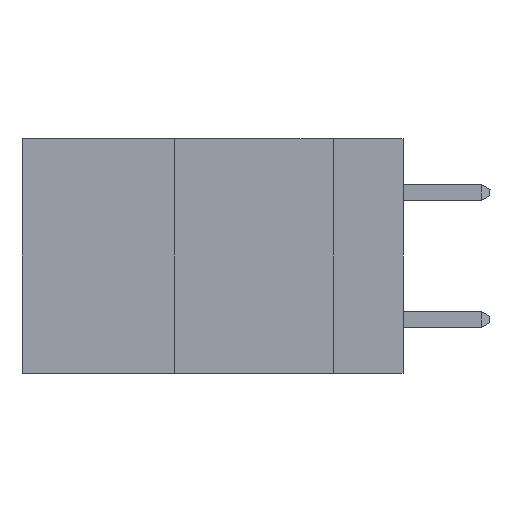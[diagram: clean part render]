
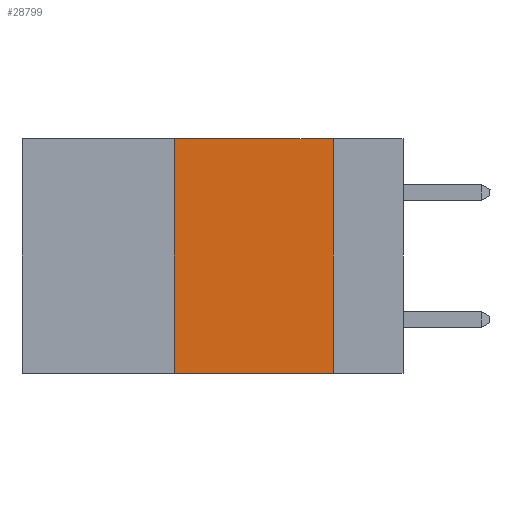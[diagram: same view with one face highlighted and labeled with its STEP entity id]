
A CAD part, left-side view. The second image highlights one B-rep face of the part: STEP entity #28799.
In plain terms, the highlighted planar face has unit normal (-1, 0, 0).
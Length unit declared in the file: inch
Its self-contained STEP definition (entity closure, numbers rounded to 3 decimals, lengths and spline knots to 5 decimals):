
#1868 = DIRECTION ( 'NONE',  ( 1., 0., 0. ) ) ;
#3075 = DIRECTION ( 'NONE',  ( 0., -1., 0. ) ) ;
#3641 = FACE_OUTER_BOUND ( 'NONE', #28108, .T. ) ;
#3772 = CARTESIAN_POINT ( 'NONE',  ( 0., 0.11, -0.37 ) ) ;
#5318 = ORIENTED_EDGE ( 'NONE', *, *, #21101, .F. ) ;
#8281 = CARTESIAN_POINT ( 'NONE',  ( 0., 0.36, -0.37 ) ) ;
#8434 = CARTESIAN_POINT ( 'NONE',  ( 0., 0.11, 0. ) ) ;
#10862 = DIRECTION ( 'NONE',  ( 0., 0., 1. ) ) ;
#11147 = CARTESIAN_POINT ( 'NONE',  ( 0., 0.36, 0. ) ) ;
#13868 = AXIS2_PLACEMENT_3D ( 'NONE', #32324, #1868, #28801 ) ;
#13940 = VECTOR ( 'NONE', #10862, 39.37008 ) ;
#14903 = EDGE_CURVE ( 'NONE', #20137, #22798, #33218, .T. ) ;
#18170 = LINE ( 'NONE', #39911, #13940 ) ;
#18423 = ORIENTED_EDGE ( 'NONE', *, *, #31303, .F. ) ;
#19138 = EDGE_CURVE ( 'NONE', #23025, #22798, #20855, .T. ) ;
#20042 = DIRECTION ( 'NONE',  ( 0., -1., 0. ) ) ;
#20137 = VERTEX_POINT ( 'NONE', #8434 ) ;
#20742 = CARTESIAN_POINT ( 'NONE',  ( 0., 0.6, -0.37 ) ) ;
#20855 = LINE ( 'NONE', #20742, #36646 ) ;
#21101 = EDGE_CURVE ( 'NONE', #23025, #32411, #18170, .T. ) ;
#22798 = VERTEX_POINT ( 'NONE', #3772 ) ;
#23025 = VERTEX_POINT ( 'NONE', #8281 ) ;
#25610 = PLANE ( 'NONE',  #13868 ) ;
#25758 = CARTESIAN_POINT ( 'NONE',  ( 0., 0.11, 0. ) ) ;
#25957 = LINE ( 'NONE', #39831, #36463 ) ;
#28108 = EDGE_LOOP ( 'NONE', ( #38353, #18423, #5318, #38404 ) ) ;
#28799 = ADVANCED_FACE ( 'NONE', ( #3641 ), #25610, .F. ) ;
#28801 = DIRECTION ( 'NONE',  ( 0., 0., -1. ) ) ;
#31108 = VECTOR ( 'NONE', #38939, 39.37008 ) ;
#31303 = EDGE_CURVE ( 'NONE', #32411, #20137, #25957, .T. ) ;
#32324 = CARTESIAN_POINT ( 'NONE',  ( 0., 0.6, 0. ) ) ;
#32411 = VERTEX_POINT ( 'NONE', #11147 ) ;
#33218 = LINE ( 'NONE', #25758, #31108 ) ;
#36463 = VECTOR ( 'NONE', #20042, 39.37008 ) ;
#36646 = VECTOR ( 'NONE', #3075, 39.37008 ) ;
#38353 = ORIENTED_EDGE ( 'NONE', *, *, #14903, .F. ) ;
#38404 = ORIENTED_EDGE ( 'NONE', *, *, #19138, .T. ) ;
#38939 = DIRECTION ( 'NONE',  ( 0., 0., -1. ) ) ;
#39831 = CARTESIAN_POINT ( 'NONE',  ( 0., 0.6, 0. ) ) ;
#39911 = CARTESIAN_POINT ( 'NONE',  ( 0., 0.36, 0. ) ) ;
